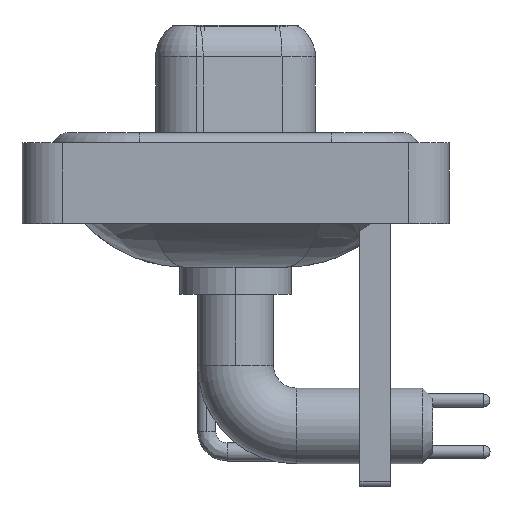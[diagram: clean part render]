
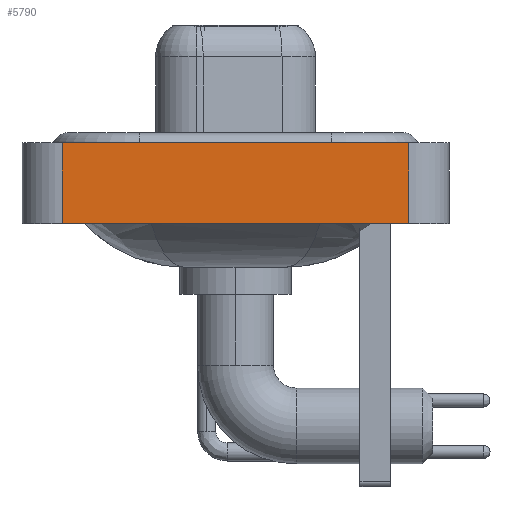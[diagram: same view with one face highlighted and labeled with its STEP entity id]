
A CAD part, left-side view. The second image highlights one B-rep face of the part: STEP entity #5790.
In plain terms, the highlighted planar face has unit normal (-1, 0, 0).
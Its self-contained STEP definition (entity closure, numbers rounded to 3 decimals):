
#93 = CARTESIAN_POINT ( 'NONE',  ( -7.35, -8.55, 0.4 ) ) ;
#325 = VECTOR ( 'NONE', #20633, 1000. ) ;
#657 = DIRECTION ( 'NONE',  ( 0., 0., 1. ) ) ;
#1394 = CARTESIAN_POINT ( 'NONE',  ( -7.35, -8.55, -3.6 ) ) ;
#3183 = PLANE ( 'NONE',  #5229 ) ;
#3700 = CARTESIAN_POINT ( 'NONE',  ( -7.35, -8.55, -3.6 ) ) ;
#4653 = CARTESIAN_POINT ( 'NONE',  ( -7.35, -8.55, -3.6 ) ) ;
#4729 = DIRECTION ( 'NONE',  ( -1., 0., 0. ) ) ;
#4817 = VERTEX_POINT ( 'NONE', #8984 ) ;
#5229 = AXIS2_PLACEMENT_3D ( 'NONE', #1394, #4729, #9465 ) ;
#5790 = ADVANCED_FACE ( 'NONE', ( #11258 ), #3183, .T. ) ;
#6405 = VECTOR ( 'NONE', #11345, 1000. ) ;
#6830 = DIRECTION ( 'NONE',  ( 0., -1., 0. ) ) ;
#6836 = EDGE_CURVE ( 'NONE', #4817, #21595, #8075, .T. ) ;
#7059 = ORIENTED_EDGE ( 'NONE', *, *, #20905, .F. ) ;
#7272 = CARTESIAN_POINT ( 'NONE',  ( -7.35, -8.55, -3.6 ) ) ;
#8075 = LINE ( 'NONE', #93, #16981 ) ;
#8984 = CARTESIAN_POINT ( 'NONE',  ( -7.35, 8.55, 0.4 ) ) ;
#9392 = ORIENTED_EDGE ( 'NONE', *, *, #6836, .F. ) ;
#9465 = DIRECTION ( 'NONE',  ( 0., 0., 1. ) ) ;
#9853 = EDGE_CURVE ( 'NONE', #11923, #14671, #18852, .T. ) ;
#11258 = FACE_OUTER_BOUND ( 'NONE', #17375, .T. ) ;
#11345 = DIRECTION ( 'NONE',  ( 0., 0., 1. ) ) ;
#11923 = VERTEX_POINT ( 'NONE', #19994 ) ;
#13068 = EDGE_CURVE ( 'NONE', #14671, #21595, #20940, .T. ) ;
#13312 = CARTESIAN_POINT ( 'NONE',  ( -7.35, -8.55, 0.4 ) ) ;
#14316 = ORIENTED_EDGE ( 'NONE', *, *, #13068, .T. ) ;
#14333 = CARTESIAN_POINT ( 'NONE',  ( -7.35, 8.55, -3.6 ) ) ;
#14671 = VERTEX_POINT ( 'NONE', #4653 ) ;
#15498 = ORIENTED_EDGE ( 'NONE', *, *, #9853, .T. ) ;
#15527 = VECTOR ( 'NONE', #657, 1000. ) ;
#16981 = VECTOR ( 'NONE', #6830, 1000. ) ;
#17375 = EDGE_LOOP ( 'NONE', ( #14316, #9392, #7059, #15498 ) ) ;
#17874 = LINE ( 'NONE', #14333, #6405 ) ;
#18852 = LINE ( 'NONE', #3700, #325 ) ;
#19994 = CARTESIAN_POINT ( 'NONE',  ( -7.35, 8.55, -3.6 ) ) ;
#20633 = DIRECTION ( 'NONE',  ( 0., -1., 0. ) ) ;
#20905 = EDGE_CURVE ( 'NONE', #11923, #4817, #17874, .T. ) ;
#20940 = LINE ( 'NONE', #7272, #15527 ) ;
#21595 = VERTEX_POINT ( 'NONE', #13312 ) ;
